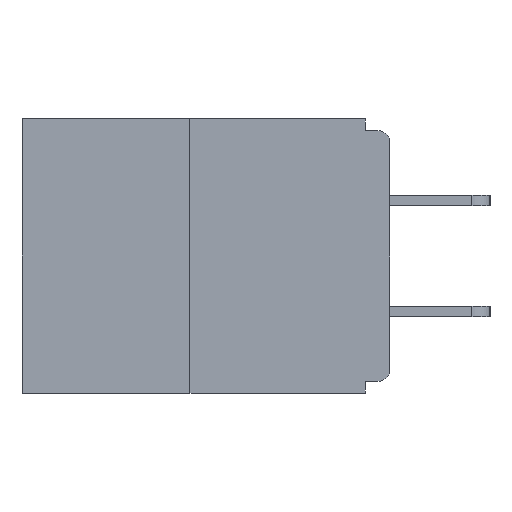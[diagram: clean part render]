
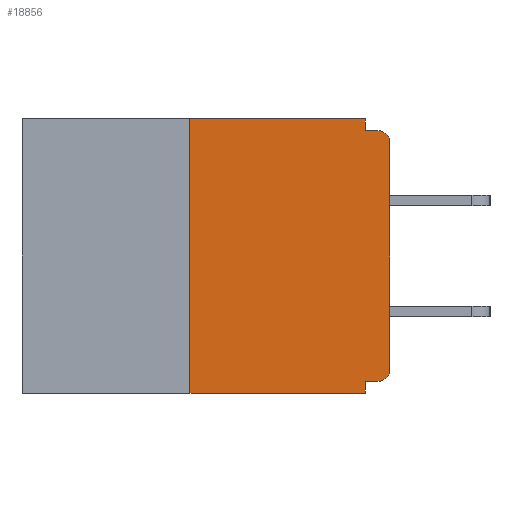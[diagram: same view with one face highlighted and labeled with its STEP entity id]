
A CAD part, left-side view. The second image highlights one B-rep face of the part: STEP entity #18856.
In plain terms, the highlighted planar face has unit normal (-1, 0, 0).
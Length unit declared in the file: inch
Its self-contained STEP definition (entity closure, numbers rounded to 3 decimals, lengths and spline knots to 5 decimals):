
#391 = DIRECTION ( 'NONE',  ( 0., 0., -1. ) ) ;
#395 = ORIENTED_EDGE ( 'NONE', *, *, #519, .T. ) ;
#519 = EDGE_CURVE ( 'NONE', #25588, #13989, #20693, .T. ) ;
#543 = VECTOR ( 'NONE', #26505, 39.37008 ) ;
#565 = CARTESIAN_POINT ( 'NONE',  ( 0., 0.031, -0.343 ) ) ;
#704 = LINE ( 'NONE', #25708, #17247 ) ;
#847 = DIRECTION ( 'NONE',  ( 0., 0., 1. ) ) ;
#1720 = ORIENTED_EDGE ( 'NONE', *, *, #4398, .F. ) ;
#1968 = CARTESIAN_POINT ( 'NONE',  ( 0., 0., -0.015 ) ) ;
#2440 = DIRECTION ( 'NONE',  ( 0., 1., 0. ) ) ;
#2889 = EDGE_CURVE ( 'NONE', #13989, #21364, #24982, .T. ) ;
#3102 = CARTESIAN_POINT ( 'NONE',  ( 0., 0.015, -0.328 ) ) ;
#3114 = EDGE_CURVE ( 'NONE', #26481, #25588, #8731, .T. ) ;
#3299 = VERTEX_POINT ( 'NONE', #13051 ) ;
#3802 = DIRECTION ( 'NONE',  ( 0., -1., 0. ) ) ;
#3994 = VERTEX_POINT ( 'NONE', #24551 ) ;
#4398 = EDGE_CURVE ( 'NONE', #26481, #20992, #11308, .T. ) ;
#4463 = EDGE_CURVE ( 'NONE', #3299, #24545, #17739, .T. ) ;
#4664 = EDGE_LOOP ( 'NONE', ( #5843, #8946, #9592, #9493, #1720, #22272, #395, #16598, #5342, #19867 ) ) ;
#4882 = CARTESIAN_POINT ( 'NONE',  ( 0., 0.46, 0. ) ) ;
#4944 = PLANE ( 'NONE',  #18761 ) ;
#5342 = ORIENTED_EDGE ( 'NONE', *, *, #23965, .F. ) ;
#5352 = CARTESIAN_POINT ( 'NONE',  ( 0., 0.46, 0. ) ) ;
#5453 = CARTESIAN_POINT ( 'NONE',  ( 0., 0.031, -0.328 ) ) ;
#5843 = ORIENTED_EDGE ( 'NONE', *, *, #14908, .F. ) ;
#5929 = VECTOR ( 'NONE', #23022, 39.37008 ) ;
#6020 = DIRECTION ( 'NONE',  ( 0., -1., 0. ) ) ;
#6663 = EDGE_CURVE ( 'NONE', #20992, #3994, #20727, .T. ) ;
#7157 = CARTESIAN_POINT ( 'NONE',  ( 0., 0.015, -0.03 ) ) ;
#7263 = DIRECTION ( 'NONE',  ( 1., 0., 0. ) ) ;
#7274 = CARTESIAN_POINT ( 'NONE',  ( 0., 0., -0.328 ) ) ;
#7770 = CARTESIAN_POINT ( 'NONE',  ( 0., 0., -0.03 ) ) ;
#8731 = CIRCLE ( 'NONE', #21585, 0.015 ) ;
#8946 = ORIENTED_EDGE ( 'NONE', *, *, #10880, .F. ) ;
#9273 = DIRECTION ( 'NONE',  ( 0., 0., -1. ) ) ;
#9467 = LINE ( 'NONE', #11483, #16758 ) ;
#9493 = ORIENTED_EDGE ( 'NONE', *, *, #6663, .F. ) ;
#9592 = ORIENTED_EDGE ( 'NONE', *, *, #11031, .T. ) ;
#9594 = DIRECTION ( 'NONE',  ( 0., -1., 0. ) ) ;
#10215 = LINE ( 'NONE', #4882, #24348 ) ;
#10880 = EDGE_CURVE ( 'NONE', #15995, #16927, #704, .T. ) ;
#11031 = EDGE_CURVE ( 'NONE', #15995, #3994, #9467, .T. ) ;
#11308 = LINE ( 'NONE', #7274, #22337 ) ;
#11483 = CARTESIAN_POINT ( 'NONE',  ( 0., 0.46, -0.343 ) ) ;
#11722 = AXIS2_PLACEMENT_3D ( 'NONE', #7157, #20309, #20186 ) ;
#12955 = CARTESIAN_POINT ( 'NONE',  ( 0., 0.25, -0.343 ) ) ;
#13051 = CARTESIAN_POINT ( 'NONE',  ( 0., 0.031, 0. ) ) ;
#13726 = DIRECTION ( 'NONE',  ( 0., 0., -1. ) ) ;
#13989 = VERTEX_POINT ( 'NONE', #7770 ) ;
#14285 = CARTESIAN_POINT ( 'NONE',  ( 0., 0., 0. ) ) ;
#14545 = CARTESIAN_POINT ( 'NONE',  ( 0., 0.25, 0. ) ) ;
#14908 = EDGE_CURVE ( 'NONE', #16927, #3299, #10215, .T. ) ;
#15168 = FACE_OUTER_BOUND ( 'NONE', #4664, .T. ) ;
#15472 = CARTESIAN_POINT ( 'NONE',  ( 0., 0.031, -0.015 ) ) ;
#15995 = VERTEX_POINT ( 'NONE', #12955 ) ;
#16598 = ORIENTED_EDGE ( 'NONE', *, *, #2889, .T. ) ;
#16758 = VECTOR ( 'NONE', #3802, 39.37008 ) ;
#16927 = VERTEX_POINT ( 'NONE', #14545 ) ;
#17247 = VECTOR ( 'NONE', #847, 39.37008 ) ;
#17555 = VECTOR ( 'NONE', #13726, 39.37008 ) ;
#17739 = LINE ( 'NONE', #24057, #17555 ) ;
#17914 = CARTESIAN_POINT ( 'NONE',  ( 0., 0.015, -0.015 ) ) ;
#18761 = AXIS2_PLACEMENT_3D ( 'NONE', #5352, #7263, #9273 ) ;
#18799 = DIRECTION ( 'NONE',  ( -1., 0., 0. ) ) ;
#18856 = ADVANCED_FACE ( 'NONE', ( #15168 ), #4944, .F. ) ;
#19867 = ORIENTED_EDGE ( 'NONE', *, *, #4463, .F. ) ;
#20186 = DIRECTION ( 'NONE',  ( 0., 0., -1. ) ) ;
#20309 = DIRECTION ( 'NONE',  ( -1., 0., 0. ) ) ;
#20693 = LINE ( 'NONE', #14285, #543 ) ;
#20727 = LINE ( 'NONE', #565, #5929 ) ;
#20992 = VERTEX_POINT ( 'NONE', #5453 ) ;
#21364 = VERTEX_POINT ( 'NONE', #17914 ) ;
#21571 = CARTESIAN_POINT ( 'NONE',  ( 0., 0., -0.313 ) ) ;
#21585 = AXIS2_PLACEMENT_3D ( 'NONE', #22985, #18799, #391 ) ;
#22272 = ORIENTED_EDGE ( 'NONE', *, *, #3114, .T. ) ;
#22337 = VECTOR ( 'NONE', #2440, 39.37008 ) ;
#22792 = VECTOR ( 'NONE', #6020, 39.37008 ) ;
#22985 = CARTESIAN_POINT ( 'NONE',  ( 0., 0.015, -0.313 ) ) ;
#23022 = DIRECTION ( 'NONE',  ( 0., 0., -1. ) ) ;
#23965 = EDGE_CURVE ( 'NONE', #24545, #21364, #24674, .T. ) ;
#24057 = CARTESIAN_POINT ( 'NONE',  ( 0., 0.031, 0. ) ) ;
#24348 = VECTOR ( 'NONE', #9594, 39.37008 ) ;
#24545 = VERTEX_POINT ( 'NONE', #15472 ) ;
#24551 = CARTESIAN_POINT ( 'NONE',  ( 0., 0.031, -0.343 ) ) ;
#24674 = LINE ( 'NONE', #1968, #22792 ) ;
#24982 = CIRCLE ( 'NONE', #11722, 0.015 ) ;
#25588 = VERTEX_POINT ( 'NONE', #21571 ) ;
#25708 = CARTESIAN_POINT ( 'NONE',  ( 0., 0.25, 0. ) ) ;
#26481 = VERTEX_POINT ( 'NONE', #3102 ) ;
#26505 = DIRECTION ( 'NONE',  ( 0., 0., 1. ) ) ;
